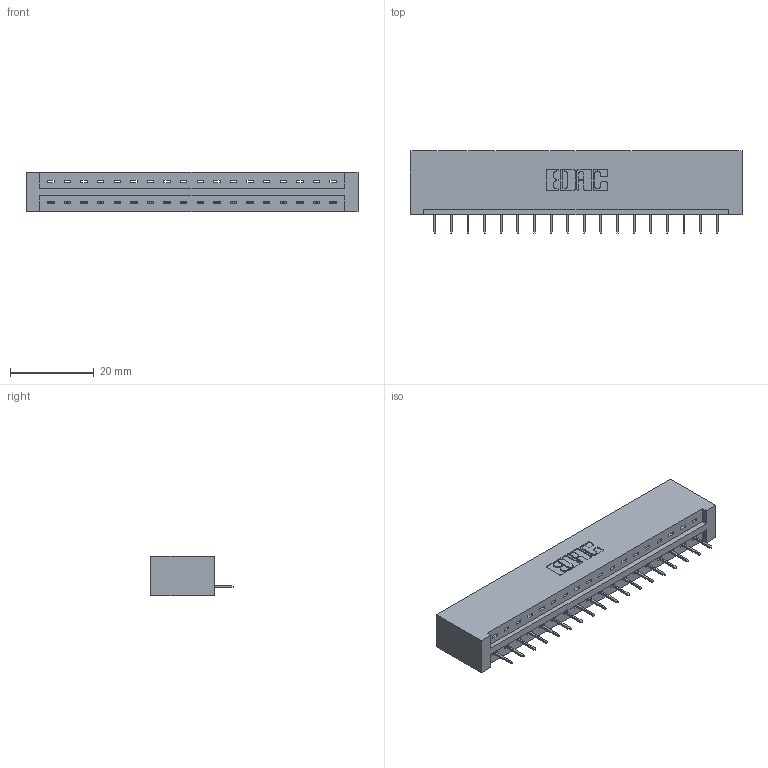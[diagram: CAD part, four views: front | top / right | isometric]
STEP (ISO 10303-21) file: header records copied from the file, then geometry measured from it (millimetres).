
FILE_DESCRIPTION (( 'STEP AP203' ), '1' );
FILE_NAME ('387-018-524-101.STEP', '2018-09-12T07:41:07', ( '' ), ( '' ), 'SwSTEP 2.0', 'SolidWorks 2016', '' );
FILE_SCHEMA (( 'CONFIG_CONTROL_DESIGN' ));
Length unit declared in the file: inch
Products named in the file (3): 337 Part_No Mounting Lugs; 345-292-001_345-293-124; 387-018-524-101
Assembly tree (19 placements, depth 2):
  387-018-524-101
    337 Part_No Mounting Lugs
    345-292-001_345-293-124  x18
Bounding box: 79.2 x 19.69 x 9.4 mm (x, y, z)
Volume: 8598.5 mm3; surface area: 8483.5 mm2
Topology: 19 solids, 19 shells, 1294 faces, 3743 edges, 2422 vertices
Faces by surface type: plane 1002, cylinder 292
Entity records: 16281 total; most frequent: CARTESIAN_POINT 2840, ORIENTED_EDGE 2794, DIRECTION 2433, EDGE_CURVE 1397, VECTOR 1281, LINE 1281, VERTEX_POINT 926, AXIS2_PLACEMENT_3D 576
